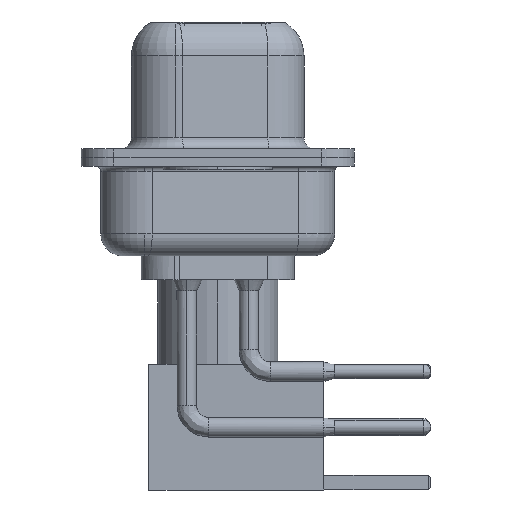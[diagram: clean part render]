
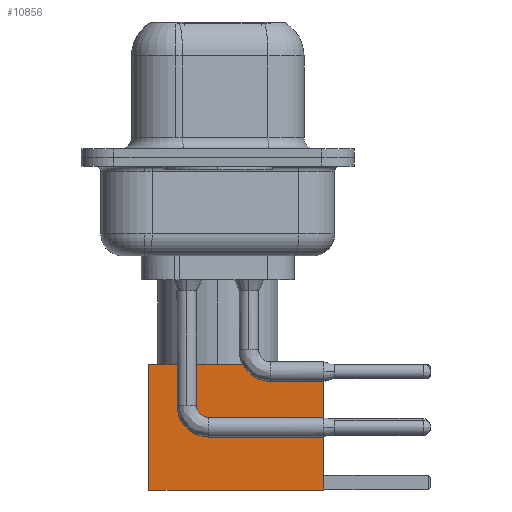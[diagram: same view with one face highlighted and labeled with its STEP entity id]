
A CAD part, left-side view. The second image highlights one B-rep face of the part: STEP entity #10856.
In plain terms, the highlighted face is planar.
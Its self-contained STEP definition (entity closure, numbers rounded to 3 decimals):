
#364 = EDGE_LOOP ( 'NONE', ( #11425, #12867, #3088, #5339 ) ) ;
#455 = VECTOR ( 'NONE', #13685, 1000. ) ;
#617 = DIRECTION ( 'NONE',  ( 0., 0., 1. ) ) ;
#1283 = CARTESIAN_POINT ( 'NONE',  ( 0., 2.875, 0. ) ) ;
#1549 = LINE ( 'NONE', #2981, #455 ) ;
#2134 = VERTEX_POINT ( 'NONE', #13808 ) ;
#2426 = AXIS2_PLACEMENT_3D ( 'NONE', #11517, #14358, #617 ) ;
#2463 = EDGE_CURVE ( 'NONE', #2134, #3577, #10765, .T. ) ;
#2981 = CARTESIAN_POINT ( 'NONE',  ( -2.875, 2.875, 0. ) ) ;
#3088 = ORIENTED_EDGE ( 'NONE', *, *, #13396, .F. ) ;
#3577 = VERTEX_POINT ( 'NONE', #13981 ) ;
#3908 = VECTOR ( 'NONE', #3989, 1000. ) ;
#3989 = DIRECTION ( 'NONE',  ( 0., 0., -1. ) ) ;
#4074 = DIRECTION ( 'NONE',  ( -1., 0., 0. ) ) ;
#4228 = VERTEX_POINT ( 'NONE', #11723 ) ;
#4492 = VECTOR ( 'NONE', #16226, 1000. ) ;
#5152 = VECTOR ( 'NONE', #4074, 1000. ) ;
#5187 = EDGE_CURVE ( 'NONE', #4228, #2134, #13523, .T. ) ;
#5339 = ORIENTED_EDGE ( 'NONE', *, *, #12553, .F. ) ;
#7016 = CARTESIAN_POINT ( 'NONE',  ( 2.875, 2.875, 0. ) ) ;
#7601 = FACE_OUTER_BOUND ( 'NONE', #364, .T. ) ;
#8159 = LINE ( 'NONE', #17573, #4492 ) ;
#10071 = CARTESIAN_POINT ( 'NONE',  ( -2.875, 2.875, 8. ) ) ;
#10765 = LINE ( 'NONE', #1283, #5152 ) ;
#10856 = ADVANCED_FACE ( 'NONE', ( #7601 ), #13037, .T. ) ;
#11425 = ORIENTED_EDGE ( 'NONE', *, *, #5187, .T. ) ;
#11517 = CARTESIAN_POINT ( 'NONE',  ( 2.875, 2.875, 0. ) ) ;
#11723 = CARTESIAN_POINT ( 'NONE',  ( 2.875, 2.875, 8. ) ) ;
#12553 = EDGE_CURVE ( 'NONE', #4228, #13023, #8159, .T. ) ;
#12867 = ORIENTED_EDGE ( 'NONE', *, *, #2463, .T. ) ;
#13023 = VERTEX_POINT ( 'NONE', #10071 ) ;
#13037 = PLANE ( 'NONE',  #2426 ) ;
#13396 = EDGE_CURVE ( 'NONE', #13023, #3577, #1549, .T. ) ;
#13523 = LINE ( 'NONE', #7016, #3908 ) ;
#13685 = DIRECTION ( 'NONE',  ( 0., 0., -1. ) ) ;
#13808 = CARTESIAN_POINT ( 'NONE',  ( 2.875, 2.875, 0. ) ) ;
#13981 = CARTESIAN_POINT ( 'NONE',  ( -2.875, 2.875, 0. ) ) ;
#14358 = DIRECTION ( 'NONE',  ( 0., 1., 0. ) ) ;
#16226 = DIRECTION ( 'NONE',  ( -1., 0., 0. ) ) ;
#17573 = CARTESIAN_POINT ( 'NONE',  ( 0., 2.875, 8. ) ) ;
